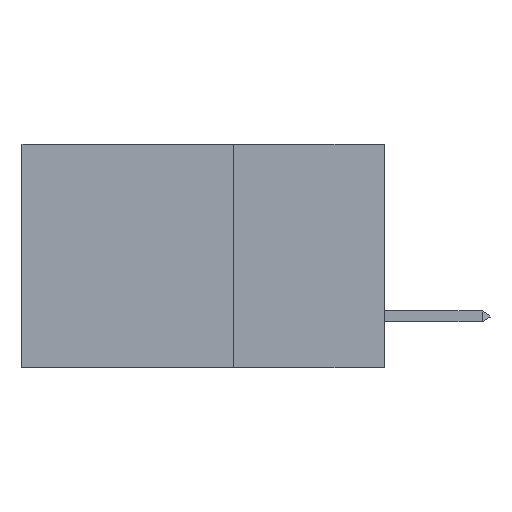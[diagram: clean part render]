
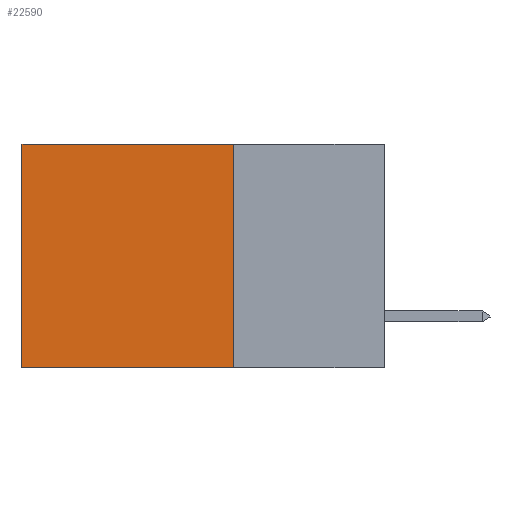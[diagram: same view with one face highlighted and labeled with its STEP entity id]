
A CAD part, left-side view. The second image highlights one B-rep face of the part: STEP entity #22590.
In plain terms, the highlighted planar face has unit normal (-1, 0, 0).
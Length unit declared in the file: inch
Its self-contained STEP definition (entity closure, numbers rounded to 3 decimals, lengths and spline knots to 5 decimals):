
#2421 = CARTESIAN_POINT ( 'NONE',  ( 0.2875, 0.25, 0. ) ) ;
#3388 = CARTESIAN_POINT ( 'NONE',  ( 0.2875, 0.25, 0. ) ) ;
#3827 = LINE ( 'NONE', #5429, #24023 ) ;
#5323 = LINE ( 'NONE', #2421, #22261 ) ;
#5429 = CARTESIAN_POINT ( 'NONE',  ( 0.2875, 0.6, 0. ) ) ;
#5831 = EDGE_CURVE ( 'NONE', #23868, #22435, #28044, .T. ) ;
#6276 = EDGE_CURVE ( 'NONE', #19543, #10426, #5323, .T. ) ;
#6625 = CARTESIAN_POINT ( 'NONE',  ( 0.2875, 0.25, 0. ) ) ;
#6965 = VECTOR ( 'NONE', #10821, 39.37008 ) ;
#9026 = EDGE_CURVE ( 'NONE', #19543, #23868, #32024, .T. ) ;
#9286 = DIRECTION ( 'NONE',  ( 1., 0., 0. ) ) ;
#10426 = VERTEX_POINT ( 'NONE', #11915 ) ;
#10821 = DIRECTION ( 'NONE',  ( 0., 1., 0. ) ) ;
#10903 = VECTOR ( 'NONE', #33354, 39.37008 ) ;
#11058 = ORIENTED_EDGE ( 'NONE', *, *, #5831, .F. ) ;
#11915 = CARTESIAN_POINT ( 'NONE',  ( 0.2875, 0.6, 0. ) ) ;
#12885 = DIRECTION ( 'NONE',  ( 0., 1., 0. ) ) ;
#16324 = CARTESIAN_POINT ( 'NONE',  ( 0.2875, 0.25, -0.37 ) ) ;
#18653 = FACE_OUTER_BOUND ( 'NONE', #25785, .T. ) ;
#19543 = VERTEX_POINT ( 'NONE', #3388 ) ;
#19577 = DIRECTION ( 'NONE',  ( 0., 0., -1. ) ) ;
#20137 = ORIENTED_EDGE ( 'NONE', *, *, #22941, .T. ) ;
#20552 = ORIENTED_EDGE ( 'NONE', *, *, #9026, .F. ) ;
#21032 = CARTESIAN_POINT ( 'NONE',  ( 0.2875, 0.25, -0.37 ) ) ;
#21929 = DIRECTION ( 'NONE',  ( 0., 0., -1. ) ) ;
#22261 = VECTOR ( 'NONE', #12885, 39.37008 ) ;
#22435 = VERTEX_POINT ( 'NONE', #23703 ) ;
#22443 = PLANE ( 'NONE',  #28405 ) ;
#22590 = ADVANCED_FACE ( 'NONE', ( #18653 ), #22443, .F. ) ;
#22941 = EDGE_CURVE ( 'NONE', #10426, #22435, #3827, .T. ) ;
#23330 = CARTESIAN_POINT ( 'NONE',  ( 0.2875, 0.25, 0. ) ) ;
#23703 = CARTESIAN_POINT ( 'NONE',  ( 0.2875, 0.6, -0.37 ) ) ;
#23868 = VERTEX_POINT ( 'NONE', #16324 ) ;
#24023 = VECTOR ( 'NONE', #21929, 39.37008 ) ;
#25785 = EDGE_LOOP ( 'NONE', ( #20137, #11058, #20552, #27935 ) ) ;
#27935 = ORIENTED_EDGE ( 'NONE', *, *, #6276, .T. ) ;
#28044 = LINE ( 'NONE', #21032, #6965 ) ;
#28405 = AXIS2_PLACEMENT_3D ( 'NONE', #6625, #9286, #19577 ) ;
#32024 = LINE ( 'NONE', #23330, #10903 ) ;
#33354 = DIRECTION ( 'NONE',  ( 0., 0., -1. ) ) ;
